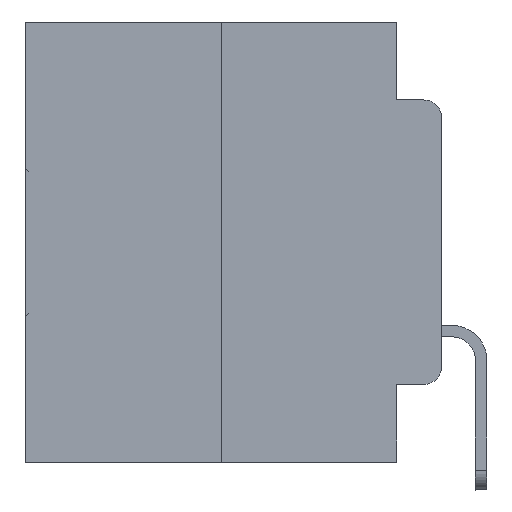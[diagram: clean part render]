
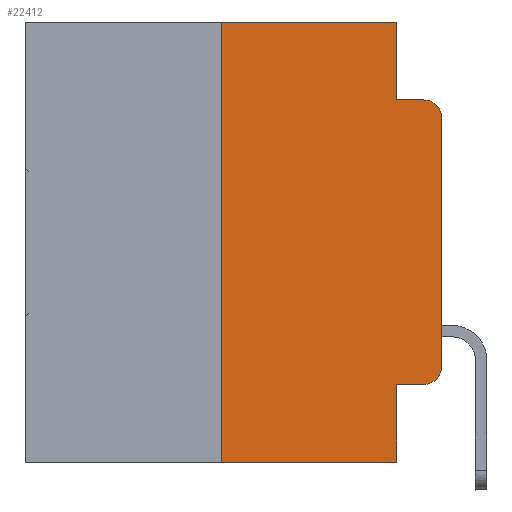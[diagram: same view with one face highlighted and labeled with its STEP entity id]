
A CAD part, left-side view. The second image highlights one B-rep face of the part: STEP entity #22412.
In plain terms, the highlighted planar face has unit normal (-1, 0, 0).
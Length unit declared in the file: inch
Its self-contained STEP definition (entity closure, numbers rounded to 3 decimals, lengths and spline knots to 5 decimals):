
#354 = ORIENTED_EDGE ( 'NONE', *, *, #25412, .F. ) ;
#1160 = LINE ( 'NONE', #15578, #10924 ) ;
#1260 = DIRECTION ( 'NONE',  ( 0., 0., 1. ) ) ;
#1264 = EDGE_LOOP ( 'NONE', ( #16542, #30570, #354, #1910, #7820, #2123, #29374, #12655, #19469, #27196 ) ) ;
#1614 = LINE ( 'NONE', #11060, #14769 ) ;
#1910 = ORIENTED_EDGE ( 'NONE', *, *, #11158, .F. ) ;
#2111 = EDGE_CURVE ( 'NONE', #22331, #7227, #1614, .T. ) ;
#2123 = ORIENTED_EDGE ( 'NONE', *, *, #2111, .F. ) ;
#2361 = LINE ( 'NONE', #14310, #26232 ) ;
#2429 = EDGE_CURVE ( 'NONE', #12780, #13831, #24417, .T. ) ;
#3920 = VECTOR ( 'NONE', #7389, 39.37008 ) ;
#4306 = VERTEX_POINT ( 'NONE', #11153 ) ;
#5221 = VERTEX_POINT ( 'NONE', #23349 ) ;
#5669 = VERTEX_POINT ( 'NONE', #13058 ) ;
#6670 = DIRECTION ( 'NONE',  ( -1., 0., 0. ) ) ;
#6712 = CARTESIAN_POINT ( 'NONE',  ( 0., 0.02, -0.4115 ) ) ;
#7227 = VERTEX_POINT ( 'NONE', #23674 ) ;
#7389 = DIRECTION ( 'NONE',  ( 0., -1., 0. ) ) ;
#7820 = ORIENTED_EDGE ( 'NONE', *, *, #9067, .F. ) ;
#8343 = VECTOR ( 'NONE', #1260, 39.37008 ) ;
#9011 = LINE ( 'NONE', #12048, #3920 ) ;
#9067 = EDGE_CURVE ( 'NONE', #7227, #12400, #2361, .T. ) ;
#9163 = AXIS2_PLACEMENT_3D ( 'NONE', #27946, #6670, #20637 ) ;
#9234 = DIRECTION ( 'NONE',  ( 0., 0., -1. ) ) ;
#9741 = EDGE_CURVE ( 'NONE', #22331, #4306, #15498, .T. ) ;
#9944 = AXIS2_PLACEMENT_3D ( 'NONE', #20011, #27312, #29944 ) ;
#10358 = VERTEX_POINT ( 'NONE', #6712 ) ;
#10838 = EDGE_CURVE ( 'NONE', #14425, #10358, #9011, .T. ) ;
#10924 = VECTOR ( 'NONE', #15269, 39.37008 ) ;
#11060 = CARTESIAN_POINT ( 'NONE',  ( 0., 0.25, 0. ) ) ;
#11153 = CARTESIAN_POINT ( 'NONE',  ( 0., 0.051, -0.5 ) ) ;
#11158 = EDGE_CURVE ( 'NONE', #12400, #5221, #21026, .T. ) ;
#11356 = DIRECTION ( 'NONE',  ( 0., 0., 1. ) ) ;
#12048 = CARTESIAN_POINT ( 'NONE',  ( 0., 0.051, -0.4115 ) ) ;
#12400 = VERTEX_POINT ( 'NONE', #25897 ) ;
#12655 = ORIENTED_EDGE ( 'NONE', *, *, #16836, .F. ) ;
#12780 = VERTEX_POINT ( 'NONE', #23787 ) ;
#13058 = CARTESIAN_POINT ( 'NONE',  ( 0., 0.02, -0.0885 ) ) ;
#13831 = VERTEX_POINT ( 'NONE', #15584 ) ;
#14254 = AXIS2_PLACEMENT_3D ( 'NONE', #22764, #25247, #25411 ) ;
#14310 = CARTESIAN_POINT ( 'NONE',  ( 0., 0.473, 0. ) ) ;
#14425 = VERTEX_POINT ( 'NONE', #29829 ) ;
#14769 = VECTOR ( 'NONE', #11356, 39.37008 ) ;
#15213 = CARTESIAN_POINT ( 'NONE',  ( 0., 0., 0. ) ) ;
#15269 = DIRECTION ( 'NONE',  ( 0., 0., -1. ) ) ;
#15338 = PLANE ( 'NONE',  #9944 ) ;
#15498 = LINE ( 'NONE', #15647, #20712 ) ;
#15578 = CARTESIAN_POINT ( 'NONE',  ( 0., 0.051, 0. ) ) ;
#15584 = CARTESIAN_POINT ( 'NONE',  ( 0., 0., -0.1085 ) ) ;
#15647 = CARTESIAN_POINT ( 'NONE',  ( 0., 0.473, -0.5 ) ) ;
#15727 = CIRCLE ( 'NONE', #14254, 0.02 ) ;
#15926 = CARTESIAN_POINT ( 'NONE',  ( 0., 0.051, -0.0885 ) ) ;
#16542 = ORIENTED_EDGE ( 'NONE', *, *, #2429, .T. ) ;
#16836 = EDGE_CURVE ( 'NONE', #14425, #4306, #1160, .T. ) ;
#17333 = VECTOR ( 'NONE', #9234, 39.37008 ) ;
#18151 = FACE_OUTER_BOUND ( 'NONE', #1264, .T. ) ;
#19469 = ORIENTED_EDGE ( 'NONE', *, *, #10838, .T. ) ;
#19785 = EDGE_CURVE ( 'NONE', #13831, #5669, #15727, .T. ) ;
#20011 = CARTESIAN_POINT ( 'NONE',  ( 0., 0.473, 0. ) ) ;
#20637 = DIRECTION ( 'NONE',  ( 0., 0., -1. ) ) ;
#20712 = VECTOR ( 'NONE', #29632, 39.37008 ) ;
#21026 = LINE ( 'NONE', #23205, #17333 ) ;
#22331 = VERTEX_POINT ( 'NONE', #27160 ) ;
#22412 = ADVANCED_FACE ( 'NONE', ( #18151 ), #15338, .F. ) ;
#22469 = DIRECTION ( 'NONE',  ( 0., -1., 0. ) ) ;
#22551 = CIRCLE ( 'NONE', #9163, 0.02 ) ;
#22764 = CARTESIAN_POINT ( 'NONE',  ( 0., 0.02, -0.1085 ) ) ;
#23205 = CARTESIAN_POINT ( 'NONE',  ( 0., 0.051, 0. ) ) ;
#23349 = CARTESIAN_POINT ( 'NONE',  ( 0., 0.051, -0.0885 ) ) ;
#23674 = CARTESIAN_POINT ( 'NONE',  ( 0., 0.25, 0. ) ) ;
#23787 = CARTESIAN_POINT ( 'NONE',  ( 0., 0., -0.3915 ) ) ;
#23913 = VECTOR ( 'NONE', #22469, 39.37008 ) ;
#23957 = DIRECTION ( 'NONE',  ( 0., -1., 0. ) ) ;
#24417 = LINE ( 'NONE', #15213, #8343 ) ;
#25247 = DIRECTION ( 'NONE',  ( -1., 0., 0. ) ) ;
#25411 = DIRECTION ( 'NONE',  ( 0., 0., -1. ) ) ;
#25412 = EDGE_CURVE ( 'NONE', #5221, #5669, #27595, .T. ) ;
#25897 = CARTESIAN_POINT ( 'NONE',  ( 0., 0.051, 0. ) ) ;
#26232 = VECTOR ( 'NONE', #23957, 39.37008 ) ;
#27160 = CARTESIAN_POINT ( 'NONE',  ( 0., 0.25, -0.5 ) ) ;
#27196 = ORIENTED_EDGE ( 'NONE', *, *, #28066, .T. ) ;
#27312 = DIRECTION ( 'NONE',  ( 1., 0., 0. ) ) ;
#27595 = LINE ( 'NONE', #15926, #23913 ) ;
#27946 = CARTESIAN_POINT ( 'NONE',  ( 0., 0.02, -0.3915 ) ) ;
#28066 = EDGE_CURVE ( 'NONE', #10358, #12780, #22551, .T. ) ;
#29374 = ORIENTED_EDGE ( 'NONE', *, *, #9741, .T. ) ;
#29632 = DIRECTION ( 'NONE',  ( 0., -1., 0. ) ) ;
#29829 = CARTESIAN_POINT ( 'NONE',  ( 0., 0.051, -0.4115 ) ) ;
#29944 = DIRECTION ( 'NONE',  ( 0., 0., -1. ) ) ;
#30570 = ORIENTED_EDGE ( 'NONE', *, *, #19785, .T. ) ;
